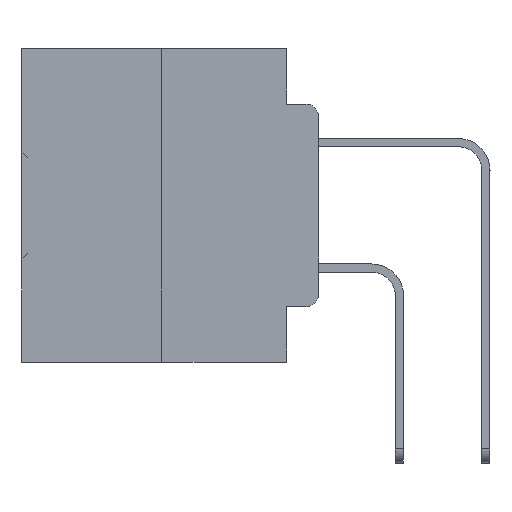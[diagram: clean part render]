
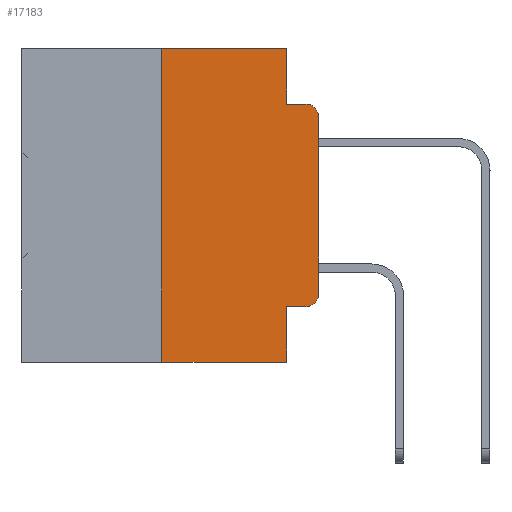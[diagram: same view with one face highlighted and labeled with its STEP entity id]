
A CAD part, left-side view. The second image highlights one B-rep face of the part: STEP entity #17183.
In plain terms, the highlighted planar face has unit normal (-1, 0, 0).
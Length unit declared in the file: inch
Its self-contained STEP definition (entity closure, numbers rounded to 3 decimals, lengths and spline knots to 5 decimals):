
#822 = CARTESIAN_POINT ( 'NONE',  ( 0., 0.473, 0. ) ) ;
#1249 = CARTESIAN_POINT ( 'NONE',  ( 0., 0.02, -0.1085 ) ) ;
#1479 = VECTOR ( 'NONE', #13171, 39.37008 ) ;
#2531 = ORIENTED_EDGE ( 'NONE', *, *, #5807, .T. ) ;
#2843 = LINE ( 'NONE', #23225, #36065 ) ;
#4304 = VECTOR ( 'NONE', #9925, 39.37008 ) ;
#5682 = EDGE_CURVE ( 'NONE', #15979, #10158, #31866, .T. ) ;
#5807 = EDGE_CURVE ( 'NONE', #10158, #20786, #27570, .T. ) ;
#5866 = EDGE_CURVE ( 'NONE', #19087, #23712, #15255, .T. ) ;
#6162 = ORIENTED_EDGE ( 'NONE', *, *, #23189, .F. ) ;
#6240 = ORIENTED_EDGE ( 'NONE', *, *, #5682, .T. ) ;
#6630 = AXIS2_PLACEMENT_3D ( 'NONE', #9193, #12242, #15974 ) ;
#6801 = CARTESIAN_POINT ( 'NONE',  ( 0., 0.25, 0. ) ) ;
#7026 = EDGE_CURVE ( 'NONE', #20786, #31282, #20342, .T. ) ;
#7162 = VERTEX_POINT ( 'NONE', #7311 ) ;
#7182 = DIRECTION ( 'NONE',  ( -1., 0., 0. ) ) ;
#7223 = LINE ( 'NONE', #23506, #10076 ) ;
#7311 = CARTESIAN_POINT ( 'NONE',  ( 0., 0.25, -0.5 ) ) ;
#7852 = ORIENTED_EDGE ( 'NONE', *, *, #18797, .F. ) ;
#8140 = DIRECTION ( 'NONE',  ( 0., 0., 1. ) ) ;
#8528 = EDGE_CURVE ( 'NONE', #27812, #31282, #28423, .T. ) ;
#8660 = LINE ( 'NONE', #25223, #10969 ) ;
#8769 = CARTESIAN_POINT ( 'NONE',  ( 0., 0.473, 0. ) ) ;
#9193 = CARTESIAN_POINT ( 'NONE',  ( 0., 0.02, -0.3915 ) ) ;
#9587 = CARTESIAN_POINT ( 'NONE',  ( 0., 0., -0.3915 ) ) ;
#9925 = DIRECTION ( 'NONE',  ( 0., -1., 0. ) ) ;
#10076 = VECTOR ( 'NONE', #30026, 39.37008 ) ;
#10158 = VERTEX_POINT ( 'NONE', #9587 ) ;
#10969 = VECTOR ( 'NONE', #25355, 39.37008 ) ;
#11563 = ORIENTED_EDGE ( 'NONE', *, *, #5866, .F. ) ;
#11678 = VERTEX_POINT ( 'NONE', #31956 ) ;
#11946 = DIRECTION ( 'NONE',  ( 1., 0., 0. ) ) ;
#12242 = DIRECTION ( 'NONE',  ( -1., 0., 0. ) ) ;
#12789 = ORIENTED_EDGE ( 'NONE', *, *, #7026, .T. ) ;
#13171 = DIRECTION ( 'NONE',  ( 0., 0., 1. ) ) ;
#13648 = CARTESIAN_POINT ( 'NONE',  ( 0., 0.02, -0.0885 ) ) ;
#15088 = EDGE_CURVE ( 'NONE', #27864, #15979, #8660, .T. ) ;
#15255 = LINE ( 'NONE', #822, #4304 ) ;
#15834 = FACE_OUTER_BOUND ( 'NONE', #34047, .T. ) ;
#15974 = DIRECTION ( 'NONE',  ( 0., 0., -1. ) ) ;
#15979 = VERTEX_POINT ( 'NONE', #17444 ) ;
#16116 = CARTESIAN_POINT ( 'NONE',  ( 0., 0., 0. ) ) ;
#16410 = CARTESIAN_POINT ( 'NONE',  ( 0., 0., -0.1085 ) ) ;
#17183 = ADVANCED_FACE ( 'NONE', ( #15834 ), #30138, .F. ) ;
#17444 = CARTESIAN_POINT ( 'NONE',  ( 0., 0.02, -0.4115 ) ) ;
#18170 = CARTESIAN_POINT ( 'NONE',  ( 0., 0.473, -0.5 ) ) ;
#18611 = AXIS2_PLACEMENT_3D ( 'NONE', #8769, #11946, #35956 ) ;
#18797 = EDGE_CURVE ( 'NONE', #7162, #19087, #2843, .T. ) ;
#18832 = DIRECTION ( 'NONE',  ( 0., 0., -1. ) ) ;
#19087 = VERTEX_POINT ( 'NONE', #6801 ) ;
#19906 = ORIENTED_EDGE ( 'NONE', *, *, #36924, .T. ) ;
#20342 = CIRCLE ( 'NONE', #27809, 0.02 ) ;
#20737 = DIRECTION ( 'NONE',  ( 0., -1., 0. ) ) ;
#20786 = VERTEX_POINT ( 'NONE', #16410 ) ;
#20829 = CARTESIAN_POINT ( 'NONE',  ( 0., 0.051, 0. ) ) ;
#21428 = LINE ( 'NONE', #20829, #27124 ) ;
#22081 = LINE ( 'NONE', #18170, #28308 ) ;
#23189 = EDGE_CURVE ( 'NONE', #27864, #11678, #21428, .T. ) ;
#23225 = CARTESIAN_POINT ( 'NONE',  ( 0., 0.25, 0. ) ) ;
#23506 = CARTESIAN_POINT ( 'NONE',  ( 0., 0.051, 0. ) ) ;
#23712 = VERTEX_POINT ( 'NONE', #29189 ) ;
#25223 = CARTESIAN_POINT ( 'NONE',  ( 0., 0.051, -0.4115 ) ) ;
#25355 = DIRECTION ( 'NONE',  ( 0., -1., 0. ) ) ;
#25865 = CARTESIAN_POINT ( 'NONE',  ( 0., 0.051, -0.0885 ) ) ;
#27124 = VECTOR ( 'NONE', #35579, 39.37008 ) ;
#27464 = VECTOR ( 'NONE', #20737, 39.37008 ) ;
#27570 = LINE ( 'NONE', #16116, #1479 ) ;
#27809 = AXIS2_PLACEMENT_3D ( 'NONE', #1249, #7182, #18832 ) ;
#27812 = VERTEX_POINT ( 'NONE', #25865 ) ;
#27864 = VERTEX_POINT ( 'NONE', #32631 ) ;
#28089 = ORIENTED_EDGE ( 'NONE', *, *, #8528, .F. ) ;
#28308 = VECTOR ( 'NONE', #37110, 39.37008 ) ;
#28423 = LINE ( 'NONE', #32951, #27464 ) ;
#29189 = CARTESIAN_POINT ( 'NONE',  ( 0., 0.051, 0. ) ) ;
#30026 = DIRECTION ( 'NONE',  ( 0., 0., -1. ) ) ;
#30138 = PLANE ( 'NONE',  #18611 ) ;
#31282 = VERTEX_POINT ( 'NONE', #13648 ) ;
#31866 = CIRCLE ( 'NONE', #6630, 0.02 ) ;
#31956 = CARTESIAN_POINT ( 'NONE',  ( 0., 0.051, -0.5 ) ) ;
#32631 = CARTESIAN_POINT ( 'NONE',  ( 0., 0.051, -0.4115 ) ) ;
#32951 = CARTESIAN_POINT ( 'NONE',  ( 0., 0.051, -0.0885 ) ) ;
#33803 = EDGE_CURVE ( 'NONE', #23712, #27812, #7223, .T. ) ;
#34047 = EDGE_LOOP ( 'NONE', ( #2531, #12789, #28089, #36908, #11563, #7852, #19906, #6162, #35842, #6240 ) ) ;
#35579 = DIRECTION ( 'NONE',  ( 0., 0., -1. ) ) ;
#35842 = ORIENTED_EDGE ( 'NONE', *, *, #15088, .T. ) ;
#35956 = DIRECTION ( 'NONE',  ( 0., 0., -1. ) ) ;
#36065 = VECTOR ( 'NONE', #8140, 39.37008 ) ;
#36908 = ORIENTED_EDGE ( 'NONE', *, *, #33803, .F. ) ;
#36924 = EDGE_CURVE ( 'NONE', #7162, #11678, #22081, .T. ) ;
#37110 = DIRECTION ( 'NONE',  ( 0., -1., 0. ) ) ;
